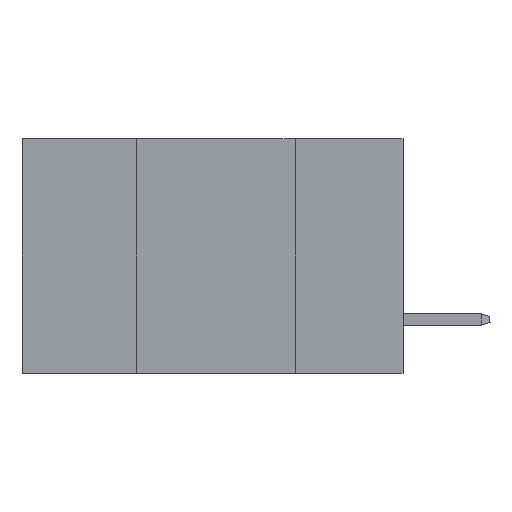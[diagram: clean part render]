
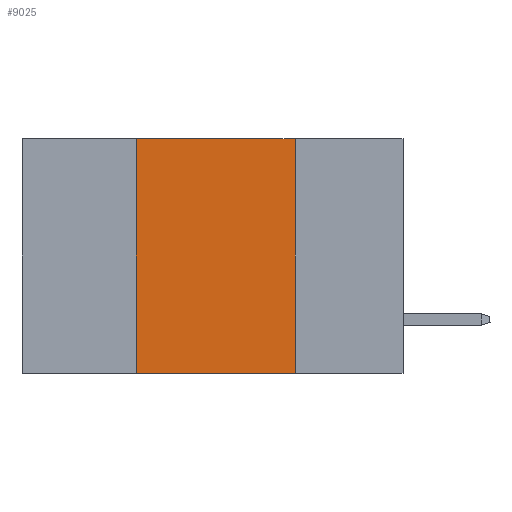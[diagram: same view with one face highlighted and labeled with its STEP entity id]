
A CAD part, left-side view. The second image highlights one B-rep face of the part: STEP entity #9025.
In plain terms, the highlighted planar face has unit normal (-1, 0, 0).
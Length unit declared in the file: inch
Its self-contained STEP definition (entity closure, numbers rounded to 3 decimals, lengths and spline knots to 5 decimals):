
#732 = AXIS2_PLACEMENT_3D ( 'NONE', #20748, #15520, #23088 ) ;
#733 = FACE_OUTER_BOUND ( 'NONE', #16960, .T. ) ;
#1257 = CARTESIAN_POINT ( 'NONE',  ( 0., 0.6, 0. ) ) ;
#1957 = EDGE_CURVE ( 'NONE', #2171, #5619, #17980, .T. ) ;
#2171 = VERTEX_POINT ( 'NONE', #20975 ) ;
#3172 = EDGE_CURVE ( 'NONE', #23021, #18172, #17167, .T. ) ;
#3181 = ORIENTED_EDGE ( 'NONE', *, *, #1957, .F. ) ;
#4280 = PLANE ( 'NONE',  #732 ) ;
#4863 = EDGE_CURVE ( 'NONE', #2171, #18172, #6340, .T. ) ;
#4955 = VECTOR ( 'NONE', #18116, 39.37008 ) ;
#5619 = VERTEX_POINT ( 'NONE', #15264 ) ;
#6340 = LINE ( 'NONE', #11705, #7687 ) ;
#7478 = CARTESIAN_POINT ( 'NONE',  ( 0., 0.17, -0.37 ) ) ;
#7687 = VECTOR ( 'NONE', #8185, 39.37008 ) ;
#8185 = DIRECTION ( 'NONE',  ( 0., -1., 0. ) ) ;
#9025 = ADVANCED_FACE ( 'NONE', ( #733 ), #4280, .F. ) ;
#10874 = ORIENTED_EDGE ( 'NONE', *, *, #3172, .F. ) ;
#11328 = VECTOR ( 'NONE', #22539, 39.37008 ) ;
#11705 = CARTESIAN_POINT ( 'NONE',  ( 0., 0.6, -0.37 ) ) ;
#12123 = LINE ( 'NONE', #1257, #20828 ) ;
#13658 = ORIENTED_EDGE ( 'NONE', *, *, #4863, .T. ) ;
#14641 = CARTESIAN_POINT ( 'NONE',  ( 0., 0.17, 0. ) ) ;
#15264 = CARTESIAN_POINT ( 'NONE',  ( 0., 0.42, 0. ) ) ;
#15520 = DIRECTION ( 'NONE',  ( 1., 0., 0. ) ) ;
#15540 = CARTESIAN_POINT ( 'NONE',  ( 0., 0.17, 0. ) ) ;
#15715 = ORIENTED_EDGE ( 'NONE', *, *, #21223, .F. ) ;
#16960 = EDGE_LOOP ( 'NONE', ( #10874, #15715, #3181, #13658 ) ) ;
#17167 = LINE ( 'NONE', #15540, #11328 ) ;
#17980 = LINE ( 'NONE', #19815, #4955 ) ;
#18116 = DIRECTION ( 'NONE',  ( 0., 0., 1. ) ) ;
#18172 = VERTEX_POINT ( 'NONE', #7478 ) ;
#19815 = CARTESIAN_POINT ( 'NONE',  ( 0., 0.42, 0. ) ) ;
#20748 = CARTESIAN_POINT ( 'NONE',  ( 0., 0.6, 0. ) ) ;
#20828 = VECTOR ( 'NONE', #22786, 39.37008 ) ;
#20975 = CARTESIAN_POINT ( 'NONE',  ( 0., 0.42, -0.37 ) ) ;
#21223 = EDGE_CURVE ( 'NONE', #5619, #23021, #12123, .T. ) ;
#22539 = DIRECTION ( 'NONE',  ( 0., 0., -1. ) ) ;
#22786 = DIRECTION ( 'NONE',  ( 0., -1., 0. ) ) ;
#23021 = VERTEX_POINT ( 'NONE', #14641 ) ;
#23088 = DIRECTION ( 'NONE',  ( 0., 0., -1. ) ) ;
